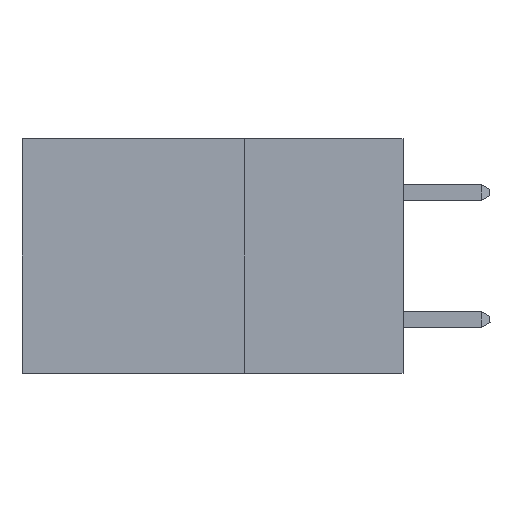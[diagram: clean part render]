
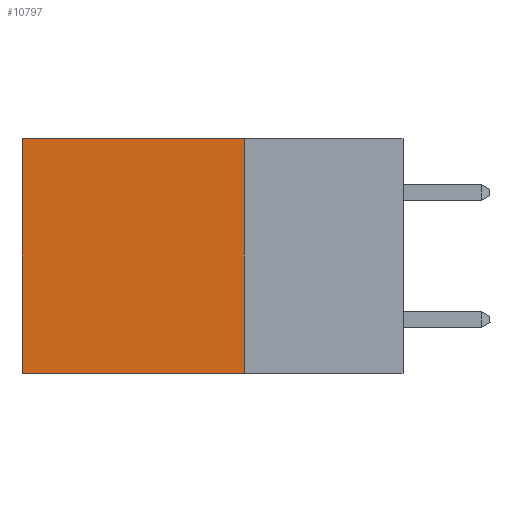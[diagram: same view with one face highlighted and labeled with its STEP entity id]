
A CAD part, left-side view. The second image highlights one B-rep face of the part: STEP entity #10797.
In plain terms, the highlighted planar face has unit normal (-1, 0, 0).
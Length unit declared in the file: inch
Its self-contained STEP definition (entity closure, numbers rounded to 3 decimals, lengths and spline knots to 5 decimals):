
#308 = VERTEX_POINT ( 'NONE', #14742 ) ;
#1562 = VERTEX_POINT ( 'NONE', #19839 ) ;
#1880 = FACE_OUTER_BOUND ( 'NONE', #9091, .T. ) ;
#4753 = VECTOR ( 'NONE', #21162, 39.37008 ) ;
#7144 = VERTEX_POINT ( 'NONE', #31737 ) ;
#7151 = AXIS2_PLACEMENT_3D ( 'NONE', #16449, #11974, #24417 ) ;
#7246 = CARTESIAN_POINT ( 'NONE',  ( 0.2875, 0.25, -0.37 ) ) ;
#7812 = VECTOR ( 'NONE', #9942, 39.37008 ) ;
#9091 = EDGE_LOOP ( 'NONE', ( #31830, #29948, #9880, #18857 ) ) ;
#9874 = EDGE_CURVE ( 'NONE', #25693, #308, #22186, .T. ) ;
#9880 = ORIENTED_EDGE ( 'NONE', *, *, #26259, .F. ) ;
#9942 = DIRECTION ( 'NONE',  ( 0., 0., -1. ) ) ;
#10797 = ADVANCED_FACE ( 'NONE', ( #1880 ), #17119, .F. ) ;
#11863 = VECTOR ( 'NONE', #24497, 39.37008 ) ;
#11974 = DIRECTION ( 'NONE',  ( 1., 0., 0. ) ) ;
#12341 = DIRECTION ( 'NONE',  ( 0., 0., -1. ) ) ;
#12661 = LINE ( 'NONE', #24940, #19995 ) ;
#13563 = EDGE_CURVE ( 'NONE', #7144, #308, #12661, .T. ) ;
#14742 = CARTESIAN_POINT ( 'NONE',  ( 0.2875, 0.6, -0.37 ) ) ;
#15080 = CARTESIAN_POINT ( 'NONE',  ( 0.2875, 0.25, 0. ) ) ;
#16449 = CARTESIAN_POINT ( 'NONE',  ( 0.2875, 0.25, 0. ) ) ;
#17119 = PLANE ( 'NONE',  #7151 ) ;
#18857 = ORIENTED_EDGE ( 'NONE', *, *, #29550, .T. ) ;
#19839 = CARTESIAN_POINT ( 'NONE',  ( 0.2875, 0.25, 0. ) ) ;
#19995 = VECTOR ( 'NONE', #12341, 39.37008 ) ;
#20356 = CARTESIAN_POINT ( 'NONE',  ( 0.2875, 0.25, -0.37 ) ) ;
#21162 = DIRECTION ( 'NONE',  ( 0., 1., 0. ) ) ;
#22186 = LINE ( 'NONE', #7246, #11863 ) ;
#22380 = CARTESIAN_POINT ( 'NONE',  ( 0.2875, 0.25, 0. ) ) ;
#22873 = LINE ( 'NONE', #22380, #7812 ) ;
#24417 = DIRECTION ( 'NONE',  ( 0., 0., -1. ) ) ;
#24497 = DIRECTION ( 'NONE',  ( 0., 1., 0. ) ) ;
#24940 = CARTESIAN_POINT ( 'NONE',  ( 0.2875, 0.6, 0. ) ) ;
#25693 = VERTEX_POINT ( 'NONE', #20356 ) ;
#26259 = EDGE_CURVE ( 'NONE', #1562, #25693, #22873, .T. ) ;
#27866 = LINE ( 'NONE', #15080, #4753 ) ;
#29550 = EDGE_CURVE ( 'NONE', #1562, #7144, #27866, .T. ) ;
#29948 = ORIENTED_EDGE ( 'NONE', *, *, #9874, .F. ) ;
#31737 = CARTESIAN_POINT ( 'NONE',  ( 0.2875, 0.6, 0. ) ) ;
#31830 = ORIENTED_EDGE ( 'NONE', *, *, #13563, .T. ) ;
